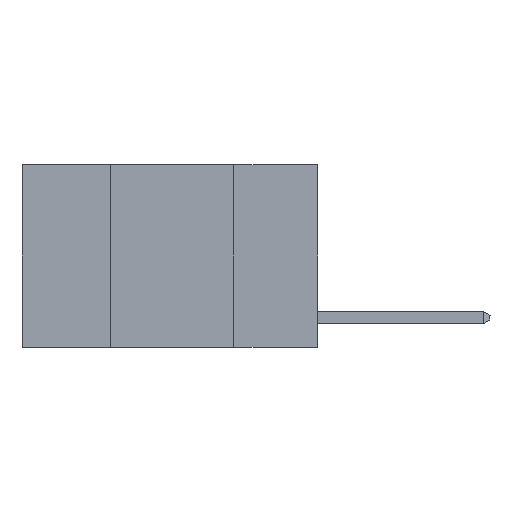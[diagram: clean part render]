
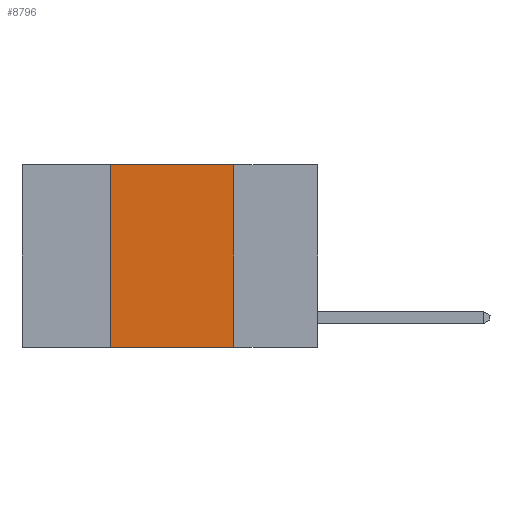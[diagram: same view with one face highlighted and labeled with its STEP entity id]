
A CAD part, left-side view. The second image highlights one B-rep face of the part: STEP entity #8796.
In plain terms, the highlighted planar face has unit normal (-1, 0, 0).
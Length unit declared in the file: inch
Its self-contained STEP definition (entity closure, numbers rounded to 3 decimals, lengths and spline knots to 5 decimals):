
#434 = CARTESIAN_POINT ( 'NONE',  ( 0., 0.17, 0. ) ) ;
#2011 = DIRECTION ( 'NONE',  ( 0., -1., 0. ) ) ;
#2056 = CARTESIAN_POINT ( 'NONE',  ( 0., 0.6, -0.37 ) ) ;
#2181 = CARTESIAN_POINT ( 'NONE',  ( 0., 0.42, 0. ) ) ;
#2924 = VERTEX_POINT ( 'NONE', #434 ) ;
#3155 = CARTESIAN_POINT ( 'NONE',  ( 0., 0.6, 0. ) ) ;
#3544 = VECTOR ( 'NONE', #7178, 39.37008 ) ;
#3704 = DIRECTION ( 'NONE',  ( 0., -1., 0. ) ) ;
#4311 = CARTESIAN_POINT ( 'NONE',  ( 0., 0.42, 0. ) ) ;
#4713 = VECTOR ( 'NONE', #2011, 39.37008 ) ;
#4932 = LINE ( 'NONE', #5089, #3544 ) ;
#5089 = CARTESIAN_POINT ( 'NONE',  ( 0., 0.17, 0. ) ) ;
#5456 = EDGE_CURVE ( 'NONE', #2924, #6032, #4932, .T. ) ;
#6020 = CARTESIAN_POINT ( 'NONE',  ( 0., 0.42, -0.37 ) ) ;
#6032 = VERTEX_POINT ( 'NONE', #9927 ) ;
#6062 = VECTOR ( 'NONE', #3704, 39.37008 ) ;
#6779 = ORIENTED_EDGE ( 'NONE', *, *, #12915, .F. ) ;
#6950 = AXIS2_PLACEMENT_3D ( 'NONE', #3155, #12287, #8331 ) ;
#7097 = EDGE_LOOP ( 'NONE', ( #11668, #6779, #8776, #9690 ) ) ;
#7178 = DIRECTION ( 'NONE',  ( 0., 0., -1. ) ) ;
#7312 = PLANE ( 'NONE',  #6950 ) ;
#7711 = EDGE_CURVE ( 'NONE', #11913, #6032, #8013, .T. ) ;
#7854 = CARTESIAN_POINT ( 'NONE',  ( 0., 0.6, 0. ) ) ;
#8013 = LINE ( 'NONE', #2056, #4713 ) ;
#8122 = LINE ( 'NONE', #7854, #6062 ) ;
#8331 = DIRECTION ( 'NONE',  ( 0., 0., -1. ) ) ;
#8451 = FACE_OUTER_BOUND ( 'NONE', #7097, .T. ) ;
#8776 = ORIENTED_EDGE ( 'NONE', *, *, #11508, .F. ) ;
#8796 = ADVANCED_FACE ( 'NONE', ( #8451 ), #7312, .F. ) ;
#9551 = VERTEX_POINT ( 'NONE', #4311 ) ;
#9623 = VECTOR ( 'NONE', #12296, 39.37008 ) ;
#9690 = ORIENTED_EDGE ( 'NONE', *, *, #7711, .T. ) ;
#9927 = CARTESIAN_POINT ( 'NONE',  ( 0., 0.17, -0.37 ) ) ;
#11508 = EDGE_CURVE ( 'NONE', #11913, #9551, #12625, .T. ) ;
#11668 = ORIENTED_EDGE ( 'NONE', *, *, #5456, .F. ) ;
#11913 = VERTEX_POINT ( 'NONE', #6020 ) ;
#12287 = DIRECTION ( 'NONE',  ( 1., 0., 0. ) ) ;
#12296 = DIRECTION ( 'NONE',  ( 0., 0., 1. ) ) ;
#12625 = LINE ( 'NONE', #2181, #9623 ) ;
#12915 = EDGE_CURVE ( 'NONE', #9551, #2924, #8122, .T. ) ;
